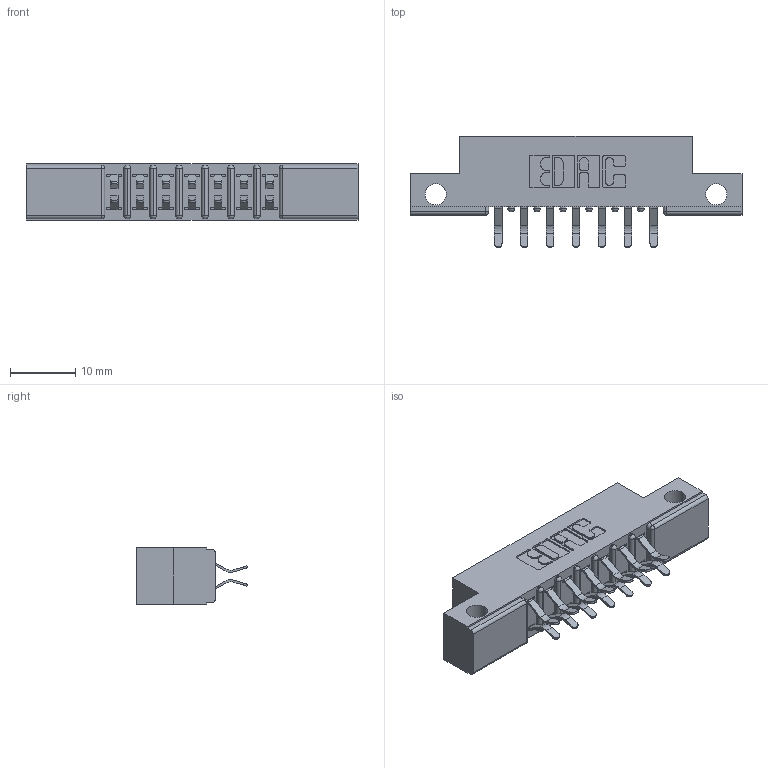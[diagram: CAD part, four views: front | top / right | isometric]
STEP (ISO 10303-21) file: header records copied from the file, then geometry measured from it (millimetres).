
FILE_DESCRIPTION (( 'STEP AP203' ), '1' );
FILE_NAME ('307-014-456-212.STEP', '2020-09-28T16:16:41', ( '' ), ( '' ), 'SwSTEP 2.0', 'SolidWorks 2020', '' );
FILE_SCHEMA (( 'CONFIG_CONTROL_DESIGN' ));
Length unit declared in the file: inch
Products named in the file (3): 307-290-001_556; 307-014-456-212; 307 Part_.128 Dia Side Mounting Holes
Assembly tree (15 placements, depth 2):
  307-014-456-212
    307 Part_.128 Dia Side Mounting Holes
    307-290-001_556  x14
Bounding box: 50.75 x 16.97 x 8.71 mm (x, y, z)
Volume: 3242.8 mm3; surface area: 4793 mm2
Topology: 15 solids, 15 shells, 826 faces, 2311 edges, 1498 vertices
Faces by surface type: plane 532, cylinder 278, sphere 16
Entity records: 10646 total; most frequent: CARTESIAN_POINT 1751, DIRECTION 1731, ORIENTED_EDGE 1730, EDGE_CURVE 865, VECTOR 647, LINE 647, VERTEX_POINT 562, AXIS2_PLACEMENT_3D 542
